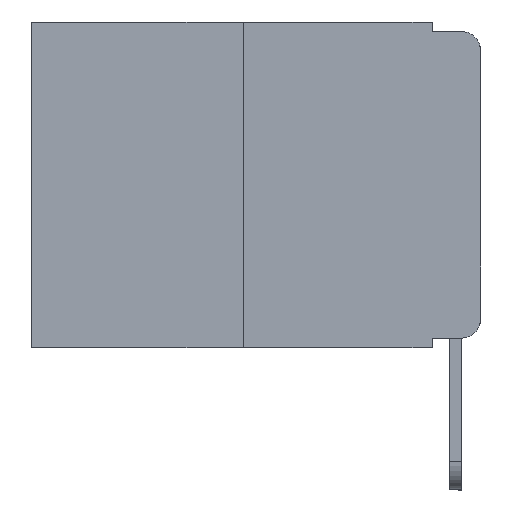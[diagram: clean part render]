
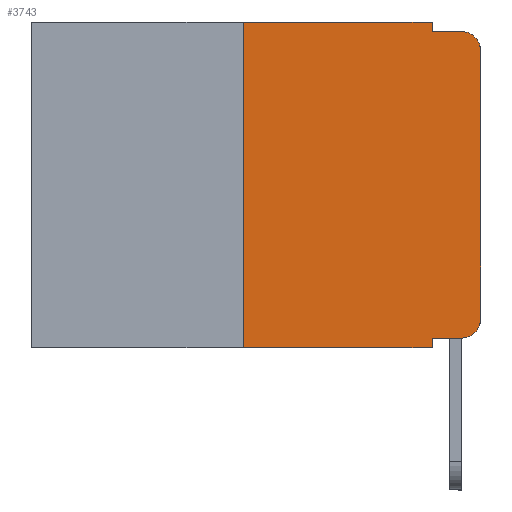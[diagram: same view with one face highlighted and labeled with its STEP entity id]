
A CAD part, left-side view. The second image highlights one B-rep face of the part: STEP entity #3743.
In plain terms, the highlighted planar face has unit normal (-1, 0, 0).
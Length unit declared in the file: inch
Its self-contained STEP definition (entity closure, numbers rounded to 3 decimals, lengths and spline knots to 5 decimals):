
#27 = VECTOR ( 'NONE', #4247, 39.37008 ) ;
#92 = LINE ( 'NONE', #5820, #1235 ) ;
#700 = DIRECTION ( 'NONE',  ( -1., 0., 0. ) ) ;
#924 = CARTESIAN_POINT ( 'NONE',  ( 0., 0.473, 0. ) ) ;
#1235 = VECTOR ( 'NONE', #14113, 39.37008 ) ;
#1437 = AXIS2_PLACEMENT_3D ( 'NONE', #16672, #10922, #8374 ) ;
#1442 = CARTESIAN_POINT ( 'NONE',  ( 0., 0.051, -0.01 ) ) ;
#1604 = CIRCLE ( 'NONE', #7306, 0.02 ) ;
#1854 = CARTESIAN_POINT ( 'NONE',  ( 0., 0.051, -0.333 ) ) ;
#1960 = VERTEX_POINT ( 'NONE', #3192 ) ;
#2445 = LINE ( 'NONE', #5645, #9546 ) ;
#2992 = CARTESIAN_POINT ( 'NONE',  ( 0., 0.051, -0.01 ) ) ;
#3192 = CARTESIAN_POINT ( 'NONE',  ( 0., 0.02, -0.333 ) ) ;
#3284 = CARTESIAN_POINT ( 'NONE',  ( 0., 0.25, 0. ) ) ;
#3525 = CIRCLE ( 'NONE', #1437, 0.02 ) ;
#3743 = ADVANCED_FACE ( 'NONE', ( #6851 ), #11185, .F. ) ;
#4083 = EDGE_CURVE ( 'NONE', #13626, #14419, #15482, .T. ) ;
#4135 = ORIENTED_EDGE ( 'NONE', *, *, #12499, .T. ) ;
#4221 = ORIENTED_EDGE ( 'NONE', *, *, #4083, .F. ) ;
#4247 = DIRECTION ( 'NONE',  ( 0., -1., 0. ) ) ;
#4428 = ORIENTED_EDGE ( 'NONE', *, *, #16478, .F. ) ;
#4645 = CARTESIAN_POINT ( 'NONE',  ( 0., 0.051, -0.333 ) ) ;
#4917 = LINE ( 'NONE', #4645, #5968 ) ;
#5004 = VERTEX_POINT ( 'NONE', #15621 ) ;
#5040 = DIRECTION ( 'NONE',  ( 0., -1., 0. ) ) ;
#5433 = DIRECTION ( 'NONE',  ( 1., 0., 0. ) ) ;
#5513 = LINE ( 'NONE', #18261, #15016 ) ;
#5546 = CARTESIAN_POINT ( 'NONE',  ( 0., 0., -0.03 ) ) ;
#5645 = CARTESIAN_POINT ( 'NONE',  ( 0., 0.051, 0. ) ) ;
#5791 = VECTOR ( 'NONE', #15311, 39.37008 ) ;
#5820 = CARTESIAN_POINT ( 'NONE',  ( 0., 0., 0. ) ) ;
#5968 = VECTOR ( 'NONE', #6069, 39.37008 ) ;
#6069 = DIRECTION ( 'NONE',  ( 0., -1., 0. ) ) ;
#6255 = EDGE_LOOP ( 'NONE', ( #4135, #16751, #4221, #16405, #4428, #12173, #15354, #13752, #10446, #7787 ) ) ;
#6414 = CARTESIAN_POINT ( 'NONE',  ( 0., 0.02, -0.313 ) ) ;
#6851 = FACE_OUTER_BOUND ( 'NONE', #6255, .T. ) ;
#6954 = CARTESIAN_POINT ( 'NONE',  ( 0., 0.051, -0.343 ) ) ;
#7005 = VECTOR ( 'NONE', #5040, 39.37008 ) ;
#7306 = AXIS2_PLACEMENT_3D ( 'NONE', #6414, #700, #15004 ) ;
#7639 = EDGE_CURVE ( 'NONE', #9768, #9471, #2445, .T. ) ;
#7787 = ORIENTED_EDGE ( 'NONE', *, *, #14870, .T. ) ;
#8063 = EDGE_CURVE ( 'NONE', #15407, #14419, #3525, .T. ) ;
#8071 = LINE ( 'NONE', #924, #7005 ) ;
#8374 = DIRECTION ( 'NONE',  ( 0., 0., -1. ) ) ;
#8675 = LINE ( 'NONE', #3284, #13793 ) ;
#8785 = EDGE_CURVE ( 'NONE', #9768, #1960, #4917, .T. ) ;
#9110 = EDGE_CURVE ( 'NONE', #9527, #5004, #8675, .T. ) ;
#9471 = VERTEX_POINT ( 'NONE', #6954 ) ;
#9527 = VERTEX_POINT ( 'NONE', #10159 ) ;
#9546 = VECTOR ( 'NONE', #11311, 39.37008 ) ;
#9563 = CARTESIAN_POINT ( 'NONE',  ( 0., 0.02, -0.01 ) ) ;
#9584 = AXIS2_PLACEMENT_3D ( 'NONE', #12512, #5433, #18084 ) ;
#9768 = VERTEX_POINT ( 'NONE', #1854 ) ;
#10159 = CARTESIAN_POINT ( 'NONE',  ( 0., 0.25, -0.343 ) ) ;
#10446 = ORIENTED_EDGE ( 'NONE', *, *, #8785, .T. ) ;
#10786 = CARTESIAN_POINT ( 'NONE',  ( 0., 0.051, 0. ) ) ;
#10922 = DIRECTION ( 'NONE',  ( -1., 0., 0. ) ) ;
#11062 = EDGE_CURVE ( 'NONE', #9527, #9471, #5513, .T. ) ;
#11185 = PLANE ( 'NONE',  #9584 ) ;
#11311 = DIRECTION ( 'NONE',  ( 0., 0., -1. ) ) ;
#11809 = CARTESIAN_POINT ( 'NONE',  ( 0., 0., -0.313 ) ) ;
#12173 = ORIENTED_EDGE ( 'NONE', *, *, #9110, .F. ) ;
#12298 = LINE ( 'NONE', #15216, #5791 ) ;
#12499 = EDGE_CURVE ( 'NONE', #13421, #15407, #92, .T. ) ;
#12512 = CARTESIAN_POINT ( 'NONE',  ( 0., 0.473, 0. ) ) ;
#13007 = DIRECTION ( 'NONE',  ( 0., 0., 1. ) ) ;
#13136 = VERTEX_POINT ( 'NONE', #10786 ) ;
#13421 = VERTEX_POINT ( 'NONE', #11809 ) ;
#13626 = VERTEX_POINT ( 'NONE', #2992 ) ;
#13752 = ORIENTED_EDGE ( 'NONE', *, *, #7639, .F. ) ;
#13793 = VECTOR ( 'NONE', #13007, 39.37008 ) ;
#13991 = DIRECTION ( 'NONE',  ( 0., -1., 0. ) ) ;
#14113 = DIRECTION ( 'NONE',  ( 0., 0., 1. ) ) ;
#14389 = EDGE_CURVE ( 'NONE', #13136, #13626, #12298, .T. ) ;
#14419 = VERTEX_POINT ( 'NONE', #9563 ) ;
#14870 = EDGE_CURVE ( 'NONE', #1960, #13421, #1604, .T. ) ;
#15004 = DIRECTION ( 'NONE',  ( 0., 0., -1. ) ) ;
#15016 = VECTOR ( 'NONE', #13991, 39.37008 ) ;
#15216 = CARTESIAN_POINT ( 'NONE',  ( 0., 0.051, 0. ) ) ;
#15311 = DIRECTION ( 'NONE',  ( 0., 0., -1. ) ) ;
#15354 = ORIENTED_EDGE ( 'NONE', *, *, #11062, .T. ) ;
#15407 = VERTEX_POINT ( 'NONE', #5546 ) ;
#15482 = LINE ( 'NONE', #1442, #27 ) ;
#15621 = CARTESIAN_POINT ( 'NONE',  ( 0., 0.25, 0. ) ) ;
#16405 = ORIENTED_EDGE ( 'NONE', *, *, #14389, .F. ) ;
#16478 = EDGE_CURVE ( 'NONE', #5004, #13136, #8071, .T. ) ;
#16672 = CARTESIAN_POINT ( 'NONE',  ( 0., 0.02, -0.03 ) ) ;
#16751 = ORIENTED_EDGE ( 'NONE', *, *, #8063, .T. ) ;
#18084 = DIRECTION ( 'NONE',  ( 0., 0., -1. ) ) ;
#18261 = CARTESIAN_POINT ( 'NONE',  ( 0., 0.473, -0.343 ) ) ;
